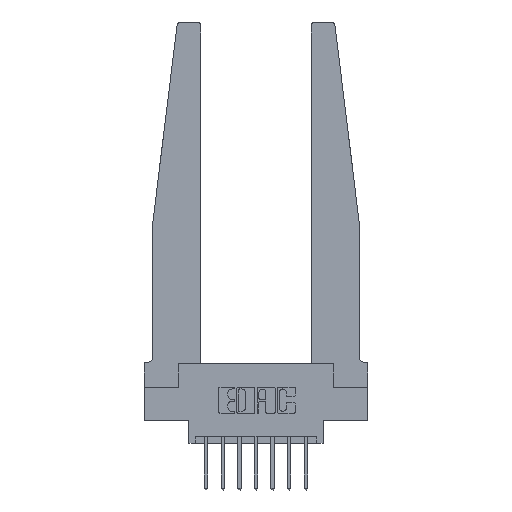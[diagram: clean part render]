
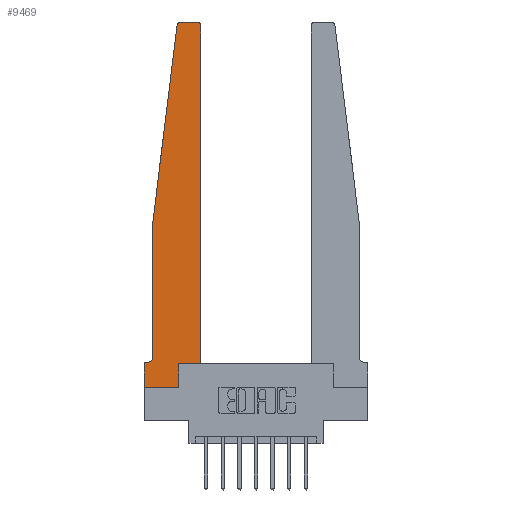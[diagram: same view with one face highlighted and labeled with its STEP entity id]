
A CAD part, top view. The second image highlights one B-rep face of the part: STEP entity #9469.
In plain terms, the highlighted planar face has unit normal (0, 0, 1).
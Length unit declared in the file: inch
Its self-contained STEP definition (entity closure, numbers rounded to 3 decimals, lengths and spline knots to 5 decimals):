
#35 = EDGE_CURVE ( 'NONE', #7224, #10468, #788, .T. ) ;
#66 = DIRECTION ( 'NONE',  ( 0., 0., 1. ) ) ;
#100 = EDGE_CURVE ( 'NONE', #9213, #8079, #2723, .T. ) ;
#260 = CARTESIAN_POINT ( 'NONE',  ( 0.015, 0.2375, 0.37 ) ) ;
#467 = ORIENTED_EDGE ( 'NONE', *, *, #35, .T. ) ;
#545 = AXIS2_PLACEMENT_3D ( 'NONE', #260, #8013, #1391 ) ;
#714 = DIRECTION ( 'NONE',  ( 1., 0., 0. ) ) ;
#788 = LINE ( 'NONE', #1524, #3415 ) ;
#812 = CARTESIAN_POINT ( 'NONE',  ( 0.065, 0.1875, 0.37 ) ) ;
#1229 = AXIS2_PLACEMENT_3D ( 'NONE', #6730, #66, #7822 ) ;
#1311 = VECTOR ( 'NONE', #1943, 39.37008 ) ;
#1391 = DIRECTION ( 'NONE',  ( -1., 0., 0. ) ) ;
#1399 = CARTESIAN_POINT ( 'NONE',  ( 0.065, 1.25, 0.37 ) ) ;
#1492 = DIRECTION ( 'NONE',  ( 0., -1., 0. ) ) ;
#1524 = CARTESIAN_POINT ( 'NONE',  ( 0.065, 1.25, 0.37 ) ) ;
#1676 = LINE ( 'NONE', #812, #1311 ) ;
#1700 = ORIENTED_EDGE ( 'NONE', *, *, #9737, .T. ) ;
#1777 = CARTESIAN_POINT ( 'NONE',  ( 0.425, 0.18, 0.37 ) ) ;
#1828 = DIRECTION ( 'NONE',  ( 1., 0., 0. ) ) ;
#1849 = CARTESIAN_POINT ( 'NONE',  ( 0., 0., 0.37 ) ) ;
#1883 = CARTESIAN_POINT ( 'NONE',  ( 0., 0.1875, 0.37 ) ) ;
#1943 = DIRECTION ( 'NONE',  ( -1., 0., 0. ) ) ;
#2175 = EDGE_CURVE ( 'NONE', #7981, #7490, #14186, .T. ) ;
#2419 = VECTOR ( 'NONE', #5641, 39.37008 ) ;
#2466 = CARTESIAN_POINT ( 'NONE',  ( 0., 0., 0.37 ) ) ;
#2587 = VECTOR ( 'NONE', #8523, 39.37008 ) ;
#2634 = CIRCLE ( 'NONE', #5979, 0.03 ) ;
#2723 = LINE ( 'NONE', #6726, #5331 ) ;
#2757 = ORIENTED_EDGE ( 'NONE', *, *, #2175, .T. ) ;
#2758 = CARTESIAN_POINT ( 'NONE',  ( 0.425, 0.18, 0.37 ) ) ;
#3111 = ORIENTED_EDGE ( 'NONE', *, *, #6220, .T. ) ;
#3415 = VECTOR ( 'NONE', #7511, 39.37008 ) ;
#3450 = ORIENTED_EDGE ( 'NONE', *, *, #6004, .T. ) ;
#3487 = DIRECTION ( 'NONE',  ( 0., 1., 0. ) ) ;
#3586 = VERTEX_POINT ( 'NONE', #9024 ) ;
#3907 = CIRCLE ( 'NONE', #545, 0.05 ) ;
#4084 = CARTESIAN_POINT ( 'NONE',  ( 0., 0.1875, 0.37 ) ) ;
#4170 = CARTESIAN_POINT ( 'NONE',  ( 0., 0., 0.37 ) ) ;
#4188 = ORIENTED_EDGE ( 'NONE', *, *, #7034, .T. ) ;
#4231 = EDGE_LOOP ( 'NONE', ( #6729, #4188, #467, #3450, #3111, #8921, #2757, #5706, #13349, #5361, #1700, #7584 ) ) ;
#4714 = EDGE_CURVE ( 'NONE', #7490, #9213, #8692, .T. ) ;
#4899 = VERTEX_POINT ( 'NONE', #2758 ) ;
#4938 = VECTOR ( 'NONE', #1492, 39.37008 ) ;
#5038 = CARTESIAN_POINT ( 'NONE',  ( 0.065, 0.2375, 0.37 ) ) ;
#5268 = AXIS2_PLACEMENT_3D ( 'NONE', #4084, #7360, #714 ) ;
#5281 = DIRECTION ( 'NONE',  ( 0., 0., 1. ) ) ;
#5331 = VECTOR ( 'NONE', #3487, 39.37008 ) ;
#5361 = ORIENTED_EDGE ( 'NONE', *, *, #8815, .T. ) ;
#5641 = DIRECTION ( 'NONE',  ( 0., 1., 0. ) ) ;
#5706 = ORIENTED_EDGE ( 'NONE', *, *, #4714, .T. ) ;
#5738 = LINE ( 'NONE', #5800, #11537 ) ;
#5745 = CARTESIAN_POINT ( 'NONE',  ( 0.24675, 2.72367, 0.37 ) ) ;
#5800 = CARTESIAN_POINT ( 'NONE',  ( 0.25, 2.75, 0.37 ) ) ;
#5979 = AXIS2_PLACEMENT_3D ( 'NONE', #11793, #5281, #12895 ) ;
#6004 = EDGE_CURVE ( 'NONE', #10468, #13354, #7821, .T. ) ;
#6220 = EDGE_CURVE ( 'NONE', #13354, #10836, #3907, .T. ) ;
#6268 = PLANE ( 'NONE',  #5268 ) ;
#6481 = CARTESIAN_POINT ( 'NONE',  ( 0.2605, 0.18, 0.37 ) ) ;
#6726 = CARTESIAN_POINT ( 'NONE',  ( 0.2605, 0.18, 0.37 ) ) ;
#6729 = ORIENTED_EDGE ( 'NONE', *, *, #9201, .T. ) ;
#6730 = CARTESIAN_POINT ( 'NONE',  ( 0.395, 2.72, 0.37 ) ) ;
#7034 = EDGE_CURVE ( 'NONE', #13839, #7224, #2634, .T. ) ;
#7224 = VERTEX_POINT ( 'NONE', #5745 ) ;
#7360 = DIRECTION ( 'NONE',  ( 0., 0., 1. ) ) ;
#7490 = VERTEX_POINT ( 'NONE', #1849 ) ;
#7511 = DIRECTION ( 'NONE',  ( -0.122, -0.992, 0. ) ) ;
#7584 = ORIENTED_EDGE ( 'NONE', *, *, #9722, .T. ) ;
#7821 = LINE ( 'NONE', #1399, #4938 ) ;
#7822 = DIRECTION ( 'NONE',  ( 1., 0., 0. ) ) ;
#7981 = VERTEX_POINT ( 'NONE', #1883 ) ;
#8013 = DIRECTION ( 'NONE',  ( 0., 0., -1. ) ) ;
#8079 = VERTEX_POINT ( 'NONE', #6481 ) ;
#8523 = DIRECTION ( 'NONE',  ( 0., -1., 0. ) ) ;
#8600 = CIRCLE ( 'NONE', #1229, 0.03 ) ;
#8692 = LINE ( 'NONE', #2466, #11263 ) ;
#8815 = EDGE_CURVE ( 'NONE', #8079, #4899, #12740, .T. ) ;
#8921 = ORIENTED_EDGE ( 'NONE', *, *, #11315, .T. ) ;
#9024 = CARTESIAN_POINT ( 'NONE',  ( 0.425, 2.72, 0.37 ) ) ;
#9037 = DIRECTION ( 'NONE',  ( 1., 0., 0. ) ) ;
#9201 = EDGE_CURVE ( 'NONE', #11817, #13839, #5738, .T. ) ;
#9213 = VERTEX_POINT ( 'NONE', #13392 ) ;
#9441 = CARTESIAN_POINT ( 'NONE',  ( 0.395, 2.75, 0.37 ) ) ;
#9469 = ADVANCED_FACE ( 'NONE', ( #11004 ), #6268, .T. ) ;
#9722 = EDGE_CURVE ( 'NONE', #3586, #11817, #8600, .T. ) ;
#9737 = EDGE_CURVE ( 'NONE', #4899, #3586, #14033, .T. ) ;
#10468 = VERTEX_POINT ( 'NONE', #13358 ) ;
#10836 = VERTEX_POINT ( 'NONE', #14180 ) ;
#11004 = FACE_OUTER_BOUND ( 'NONE', #4231, .T. ) ;
#11010 = CARTESIAN_POINT ( 'NONE',  ( 0.425, 0.18, 0.37 ) ) ;
#11263 = VECTOR ( 'NONE', #9037, 39.37008 ) ;
#11315 = EDGE_CURVE ( 'NONE', #10836, #7981, #1676, .T. ) ;
#11537 = VECTOR ( 'NONE', #13443, 39.37008 ) ;
#11793 = CARTESIAN_POINT ( 'NONE',  ( 0.27653, 2.72, 0.37 ) ) ;
#11817 = VERTEX_POINT ( 'NONE', #9441 ) ;
#12397 = VECTOR ( 'NONE', #1828, 39.37008 ) ;
#12601 = CARTESIAN_POINT ( 'NONE',  ( 0.27653, 2.75, 0.37 ) ) ;
#12740 = LINE ( 'NONE', #1777, #12397 ) ;
#12895 = DIRECTION ( 'NONE',  ( 1., 0., 0. ) ) ;
#13349 = ORIENTED_EDGE ( 'NONE', *, *, #100, .T. ) ;
#13354 = VERTEX_POINT ( 'NONE', #5038 ) ;
#13358 = CARTESIAN_POINT ( 'NONE',  ( 0.065, 1.25, 0.37 ) ) ;
#13392 = CARTESIAN_POINT ( 'NONE',  ( 0.2605, 0., 0.37 ) ) ;
#13443 = DIRECTION ( 'NONE',  ( -1., 0., 0. ) ) ;
#13839 = VERTEX_POINT ( 'NONE', #12601 ) ;
#14033 = LINE ( 'NONE', #11010, #2419 ) ;
#14180 = CARTESIAN_POINT ( 'NONE',  ( 0.015, 0.1875, 0.37 ) ) ;
#14186 = LINE ( 'NONE', #4170, #2587 ) ;
